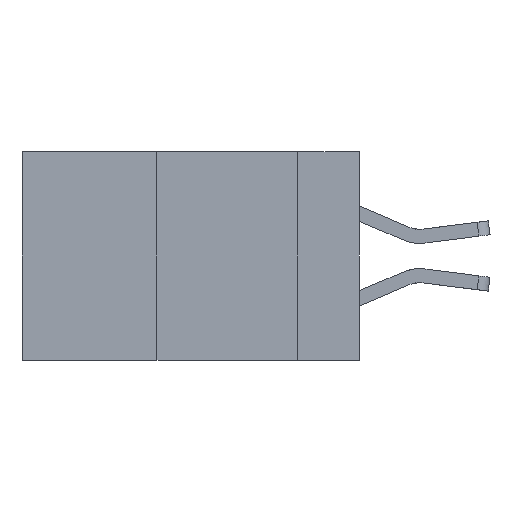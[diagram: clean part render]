
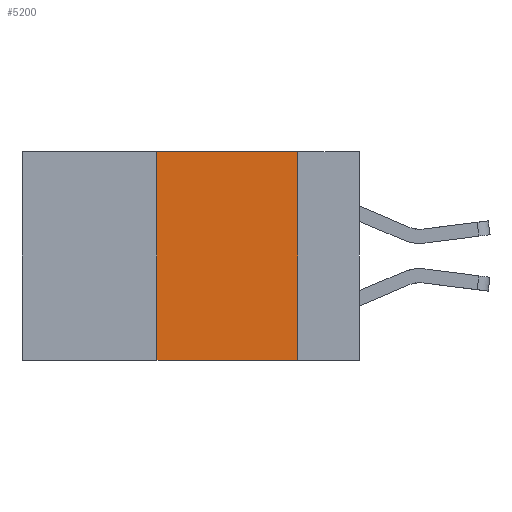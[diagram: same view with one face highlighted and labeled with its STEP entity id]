
A CAD part, left-side view. The second image highlights one B-rep face of the part: STEP entity #5200.
In plain terms, the highlighted planar face has unit normal (-1, 0, 0).
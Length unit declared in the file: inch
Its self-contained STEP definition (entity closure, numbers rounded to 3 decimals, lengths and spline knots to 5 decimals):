
#256 = DIRECTION ( 'NONE',  ( 0., -1., 0. ) ) ;
#327 = CARTESIAN_POINT ( 'NONE',  ( 0., 0.6, 0. ) ) ;
#664 = LINE ( 'NONE', #11290, #13131 ) ;
#1992 = ORIENTED_EDGE ( 'NONE', *, *, #6878, .T. ) ;
#2150 = VECTOR ( 'NONE', #7022, 39.37008 ) ;
#2361 = LINE ( 'NONE', #14483, #15184 ) ;
#3049 = VERTEX_POINT ( 'NONE', #5553 ) ;
#3548 = EDGE_CURVE ( 'NONE', #3049, #12975, #5199, .T. ) ;
#3825 = VERTEX_POINT ( 'NONE', #3909 ) ;
#3909 = CARTESIAN_POINT ( 'NONE',  ( 0., 0.36, -0.37 ) ) ;
#4097 = VERTEX_POINT ( 'NONE', #13900 ) ;
#5199 = LINE ( 'NONE', #327, #7562 ) ;
#5200 = ADVANCED_FACE ( 'NONE', ( #7535 ), #14193, .F. ) ;
#5553 = CARTESIAN_POINT ( 'NONE',  ( 0., 0.36, 0. ) ) ;
#5862 = CARTESIAN_POINT ( 'NONE',  ( 0., 0.36, 0. ) ) ;
#6182 = EDGE_LOOP ( 'NONE', ( #13981, #13258, #13801, #1992 ) ) ;
#6799 = EDGE_CURVE ( 'NONE', #12975, #4097, #664, .T. ) ;
#6878 = EDGE_CURVE ( 'NONE', #3825, #4097, #2361, .T. ) ;
#7022 = DIRECTION ( 'NONE',  ( 0., 0., 1. ) ) ;
#7535 = FACE_OUTER_BOUND ( 'NONE', #6182, .T. ) ;
#7562 = VECTOR ( 'NONE', #256, 39.37008 ) ;
#8351 = LINE ( 'NONE', #5862, #2150 ) ;
#9417 = CARTESIAN_POINT ( 'NONE',  ( 0., 0.6, 0. ) ) ;
#9764 = CARTESIAN_POINT ( 'NONE',  ( 0., 0.11, 0. ) ) ;
#10941 = EDGE_CURVE ( 'NONE', #3825, #3049, #8351, .T. ) ;
#11290 = CARTESIAN_POINT ( 'NONE',  ( 0., 0.11, 0. ) ) ;
#12769 = DIRECTION ( 'NONE',  ( 0., 0., -1. ) ) ;
#12771 = DIRECTION ( 'NONE',  ( 1., 0., 0. ) ) ;
#12831 = DIRECTION ( 'NONE',  ( 0., -1., 0. ) ) ;
#12975 = VERTEX_POINT ( 'NONE', #9764 ) ;
#13120 = DIRECTION ( 'NONE',  ( 0., 0., -1. ) ) ;
#13131 = VECTOR ( 'NONE', #13120, 39.37008 ) ;
#13258 = ORIENTED_EDGE ( 'NONE', *, *, #3548, .F. ) ;
#13801 = ORIENTED_EDGE ( 'NONE', *, *, #10941, .F. ) ;
#13900 = CARTESIAN_POINT ( 'NONE',  ( 0., 0.11, -0.37 ) ) ;
#13981 = ORIENTED_EDGE ( 'NONE', *, *, #6799, .F. ) ;
#14193 = PLANE ( 'NONE',  #14648 ) ;
#14483 = CARTESIAN_POINT ( 'NONE',  ( 0., 0.6, -0.37 ) ) ;
#14648 = AXIS2_PLACEMENT_3D ( 'NONE', #9417, #12771, #12769 ) ;
#15184 = VECTOR ( 'NONE', #12831, 39.37008 ) ;
